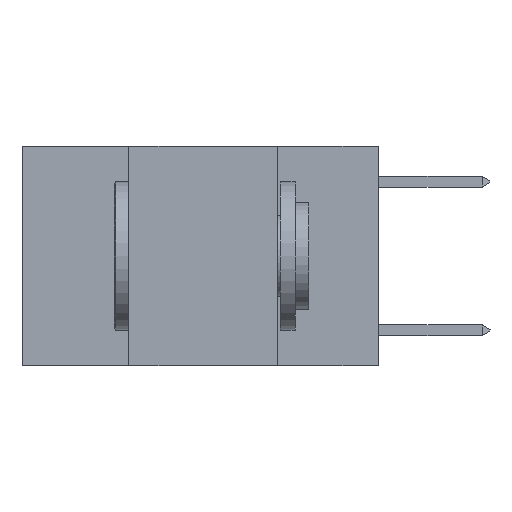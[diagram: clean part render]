
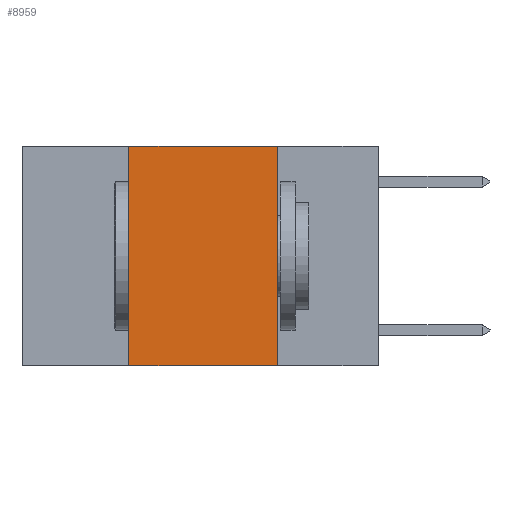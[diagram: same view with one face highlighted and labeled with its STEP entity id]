
A CAD part, left-side view. The second image highlights one B-rep face of the part: STEP entity #8959.
In plain terms, the highlighted planar face has unit normal (-1, 0, 0).
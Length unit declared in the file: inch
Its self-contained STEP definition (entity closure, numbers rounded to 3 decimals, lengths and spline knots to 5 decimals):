
#1193 = VERTEX_POINT ( 'NONE', #16141 ) ;
#2196 = VERTEX_POINT ( 'NONE', #18148 ) ;
#2263 = DIRECTION ( 'NONE',  ( 0., -1., 0. ) ) ;
#2648 = EDGE_CURVE ( 'NONE', #8821, #17796, #19472, .T. ) ;
#3189 = VECTOR ( 'NONE', #10910, 39.37008 ) ;
#3268 = ORIENTED_EDGE ( 'NONE', *, *, #14088, .F. ) ;
#4946 = ORIENTED_EDGE ( 'NONE', *, *, #2648, .F. ) ;
#5281 = CARTESIAN_POINT ( 'NONE',  ( 0., 0.6, 0. ) ) ;
#5331 = CARTESIAN_POINT ( 'NONE',  ( 0., 0.17, 0. ) ) ;
#8455 = CARTESIAN_POINT ( 'NONE',  ( 0., 0.6, 0. ) ) ;
#8765 = CARTESIAN_POINT ( 'NONE',  ( 0., 0.42, 0. ) ) ;
#8821 = VERTEX_POINT ( 'NONE', #8765 ) ;
#8959 = ADVANCED_FACE ( 'NONE', ( #13427 ), #17967, .F. ) ;
#9602 = ORIENTED_EDGE ( 'NONE', *, *, #12781, .T. ) ;
#10072 = VECTOR ( 'NONE', #11631, 39.37008 ) ;
#10292 = CARTESIAN_POINT ( 'NONE',  ( 0., 0.6, -0.37 ) ) ;
#10910 = DIRECTION ( 'NONE',  ( 0., 0., -1. ) ) ;
#11483 = DIRECTION ( 'NONE',  ( 1., 0., 0. ) ) ;
#11578 = LINE ( 'NONE', #14848, #20322 ) ;
#11631 = DIRECTION ( 'NONE',  ( 0., -1., 0. ) ) ;
#12544 = LINE ( 'NONE', #17207, #3189 ) ;
#12781 = EDGE_CURVE ( 'NONE', #2196, #1193, #19689, .T. ) ;
#13427 = FACE_OUTER_BOUND ( 'NONE', #18346, .T. ) ;
#14088 = EDGE_CURVE ( 'NONE', #2196, #8821, #11578, .T. ) ;
#14848 = CARTESIAN_POINT ( 'NONE',  ( 0., 0.42, 0. ) ) ;
#15598 = ORIENTED_EDGE ( 'NONE', *, *, #18867, .F. ) ;
#16141 = CARTESIAN_POINT ( 'NONE',  ( 0., 0.17, -0.37 ) ) ;
#17207 = CARTESIAN_POINT ( 'NONE',  ( 0., 0.17, 0. ) ) ;
#17796 = VERTEX_POINT ( 'NONE', #5331 ) ;
#17967 = PLANE ( 'NONE',  #19655 ) ;
#18070 = DIRECTION ( 'NONE',  ( 0., 0., 1. ) ) ;
#18148 = CARTESIAN_POINT ( 'NONE',  ( 0., 0.42, -0.37 ) ) ;
#18346 = EDGE_LOOP ( 'NONE', ( #15598, #4946, #3268, #9602 ) ) ;
#18867 = EDGE_CURVE ( 'NONE', #17796, #1193, #12544, .T. ) ;
#19294 = VECTOR ( 'NONE', #2263, 39.37008 ) ;
#19472 = LINE ( 'NONE', #5281, #10072 ) ;
#19655 = AXIS2_PLACEMENT_3D ( 'NONE', #8455, #11483, #19727 ) ;
#19689 = LINE ( 'NONE', #10292, #19294 ) ;
#19727 = DIRECTION ( 'NONE',  ( 0., 0., -1. ) ) ;
#20322 = VECTOR ( 'NONE', #18070, 39.37008 ) ;
